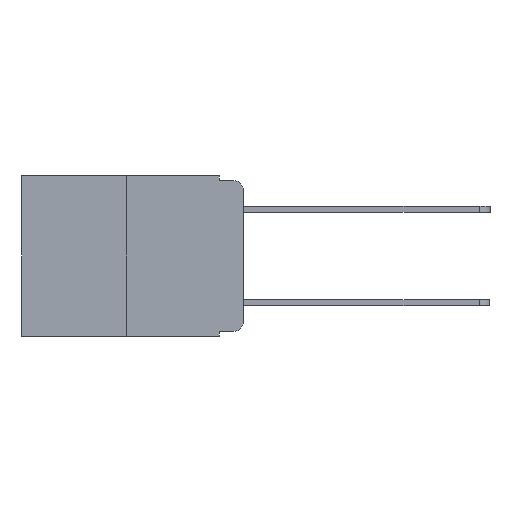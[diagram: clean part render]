
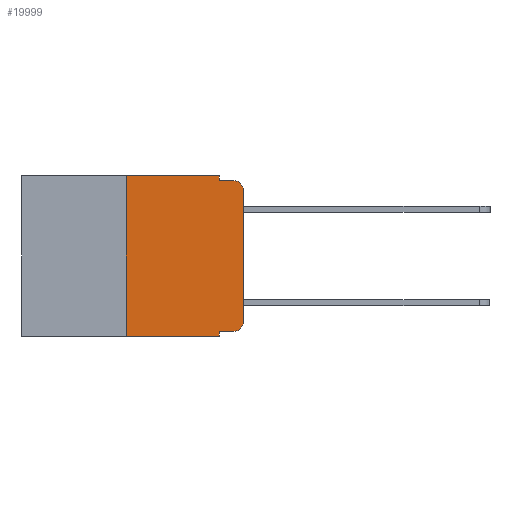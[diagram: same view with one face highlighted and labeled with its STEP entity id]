
A CAD part, left-side view. The second image highlights one B-rep face of the part: STEP entity #19999.
In plain terms, the highlighted planar face has unit normal (-1, 0, 0).
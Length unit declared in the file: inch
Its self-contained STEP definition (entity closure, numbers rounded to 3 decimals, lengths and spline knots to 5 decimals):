
#304 = EDGE_CURVE ( 'NONE', #18079, #22471, #24202, .T. ) ;
#1035 = VERTEX_POINT ( 'NONE', #6593 ) ;
#1278 = EDGE_CURVE ( 'NONE', #17911, #11037, #3124, .T. ) ;
#1807 = ORIENTED_EDGE ( 'NONE', *, *, #4144, .F. ) ;
#1869 = EDGE_CURVE ( 'NONE', #8268, #23707, #19609, .T. ) ;
#2093 = DIRECTION ( 'NONE',  ( -1., 0., 0. ) ) ;
#2181 = CARTESIAN_POINT ( 'NONE',  ( 0., 0.473, -0.343 ) ) ;
#2718 = CIRCLE ( 'NONE', #12127, 0.02 ) ;
#2854 = VECTOR ( 'NONE', #23391, 39.37008 ) ;
#2935 = DIRECTION ( 'NONE',  ( -1., 0., 0. ) ) ;
#3124 = LINE ( 'NONE', #20350, #7604 ) ;
#3215 = VECTOR ( 'NONE', #23622, 39.37008 ) ;
#3703 = CARTESIAN_POINT ( 'NONE',  ( 0., 0.02, -0.333 ) ) ;
#3966 = EDGE_CURVE ( 'NONE', #18859, #23014, #7691, .T. ) ;
#4131 = LINE ( 'NONE', #21237, #18024 ) ;
#4144 = EDGE_CURVE ( 'NONE', #11037, #8268, #19715, .T. ) ;
#4169 = CARTESIAN_POINT ( 'NONE',  ( 0., 0., -0.03 ) ) ;
#4577 = VECTOR ( 'NONE', #20087, 39.37008 ) ;
#4980 = CARTESIAN_POINT ( 'NONE',  ( 0., 0.02, -0.01 ) ) ;
#5814 = CARTESIAN_POINT ( 'NONE',  ( 0., 0.051, -0.343 ) ) ;
#5828 = EDGE_CURVE ( 'NONE', #1035, #7063, #7940, .T. ) ;
#6150 = CARTESIAN_POINT ( 'NONE',  ( 0., 0.473, 0. ) ) ;
#6231 = DIRECTION ( 'NONE',  ( 1., 0., 0. ) ) ;
#6593 = CARTESIAN_POINT ( 'NONE',  ( 0., 0., -0.313 ) ) ;
#6726 = ORIENTED_EDGE ( 'NONE', *, *, #1278, .F. ) ;
#7063 = VERTEX_POINT ( 'NONE', #4169 ) ;
#7154 = CARTESIAN_POINT ( 'NONE',  ( 0., 0.051, 0. ) ) ;
#7604 = VECTOR ( 'NONE', #22172, 39.37008 ) ;
#7691 = LINE ( 'NONE', #10705, #3215 ) ;
#7940 = LINE ( 'NONE', #16113, #2854 ) ;
#8268 = VERTEX_POINT ( 'NONE', #13368 ) ;
#8592 = EDGE_CURVE ( 'NONE', #7063, #23707, #2718, .T. ) ;
#8645 = ORIENTED_EDGE ( 'NONE', *, *, #9179, .F. ) ;
#8904 = CARTESIAN_POINT ( 'NONE',  ( 0., 0.051, -0.01 ) ) ;
#9179 = EDGE_CURVE ( 'NONE', #18859, #22471, #9871, .T. ) ;
#9273 = VECTOR ( 'NONE', #13228, 39.37008 ) ;
#9871 = LINE ( 'NONE', #24201, #9273 ) ;
#10705 = CARTESIAN_POINT ( 'NONE',  ( 0., 0.051, -0.333 ) ) ;
#11033 = AXIS2_PLACEMENT_3D ( 'NONE', #6150, #6231, #19390 ) ;
#11037 = VERTEX_POINT ( 'NONE', #7154 ) ;
#11125 = DIRECTION ( 'NONE',  ( 0., 0., -1. ) ) ;
#11912 = PLANE ( 'NONE',  #11033 ) ;
#12127 = AXIS2_PLACEMENT_3D ( 'NONE', #14324, #2935, #16182 ) ;
#13102 = EDGE_CURVE ( 'NONE', #23014, #1035, #17752, .T. ) ;
#13228 = DIRECTION ( 'NONE',  ( 0., 0., -1. ) ) ;
#13271 = EDGE_CURVE ( 'NONE', #18079, #17911, #4131, .T. ) ;
#13368 = CARTESIAN_POINT ( 'NONE',  ( 0., 0.051, -0.01 ) ) ;
#13425 = ORIENTED_EDGE ( 'NONE', *, *, #13271, .F. ) ;
#13516 = CARTESIAN_POINT ( 'NONE',  ( 0., 0.02, -0.313 ) ) ;
#13597 = DIRECTION ( 'NONE',  ( 0., -1., 0. ) ) ;
#14265 = EDGE_LOOP ( 'NONE', ( #17552, #19815, #20511, #1807, #6726, #13425, #16540, #8645, #22713, #15420 ) ) ;
#14324 = CARTESIAN_POINT ( 'NONE',  ( 0., 0.02, -0.03 ) ) ;
#15387 = DIRECTION ( 'NONE',  ( 0., 0., -1. ) ) ;
#15420 = ORIENTED_EDGE ( 'NONE', *, *, #13102, .T. ) ;
#16113 = CARTESIAN_POINT ( 'NONE',  ( 0., 0., 0. ) ) ;
#16182 = DIRECTION ( 'NONE',  ( 0., 0., -1. ) ) ;
#16540 = ORIENTED_EDGE ( 'NONE', *, *, #304, .T. ) ;
#17552 = ORIENTED_EDGE ( 'NONE', *, *, #5828, .T. ) ;
#17752 = CIRCLE ( 'NONE', #20879, 0.02 ) ;
#17911 = VERTEX_POINT ( 'NONE', #18352 ) ;
#18024 = VECTOR ( 'NONE', #23071, 39.37008 ) ;
#18079 = VERTEX_POINT ( 'NONE', #18909 ) ;
#18235 = VECTOR ( 'NONE', #13597, 39.37008 ) ;
#18352 = CARTESIAN_POINT ( 'NONE',  ( 0., 0.25, 0. ) ) ;
#18859 = VERTEX_POINT ( 'NONE', #19598 ) ;
#18909 = CARTESIAN_POINT ( 'NONE',  ( 0., 0.25, -0.343 ) ) ;
#19390 = DIRECTION ( 'NONE',  ( 0., 0., -1. ) ) ;
#19598 = CARTESIAN_POINT ( 'NONE',  ( 0., 0.051, -0.333 ) ) ;
#19609 = LINE ( 'NONE', #8904, #4577 ) ;
#19715 = LINE ( 'NONE', #20376, #23965 ) ;
#19815 = ORIENTED_EDGE ( 'NONE', *, *, #8592, .T. ) ;
#19999 = ADVANCED_FACE ( 'NONE', ( #22957 ), #11912, .F. ) ;
#20087 = DIRECTION ( 'NONE',  ( 0., -1., 0. ) ) ;
#20350 = CARTESIAN_POINT ( 'NONE',  ( 0., 0.473, 0. ) ) ;
#20376 = CARTESIAN_POINT ( 'NONE',  ( 0., 0.051, 0. ) ) ;
#20511 = ORIENTED_EDGE ( 'NONE', *, *, #1869, .F. ) ;
#20879 = AXIS2_PLACEMENT_3D ( 'NONE', #13516, #2093, #15387 ) ;
#21237 = CARTESIAN_POINT ( 'NONE',  ( 0., 0.25, 0. ) ) ;
#22172 = DIRECTION ( 'NONE',  ( 0., -1., 0. ) ) ;
#22471 = VERTEX_POINT ( 'NONE', #5814 ) ;
#22713 = ORIENTED_EDGE ( 'NONE', *, *, #3966, .T. ) ;
#22957 = FACE_OUTER_BOUND ( 'NONE', #14265, .T. ) ;
#23014 = VERTEX_POINT ( 'NONE', #3703 ) ;
#23071 = DIRECTION ( 'NONE',  ( 0., 0., 1. ) ) ;
#23391 = DIRECTION ( 'NONE',  ( 0., 0., 1. ) ) ;
#23622 = DIRECTION ( 'NONE',  ( 0., -1., 0. ) ) ;
#23707 = VERTEX_POINT ( 'NONE', #4980 ) ;
#23965 = VECTOR ( 'NONE', #11125, 39.37008 ) ;
#24201 = CARTESIAN_POINT ( 'NONE',  ( 0., 0.051, 0. ) ) ;
#24202 = LINE ( 'NONE', #2181, #18235 ) ;
